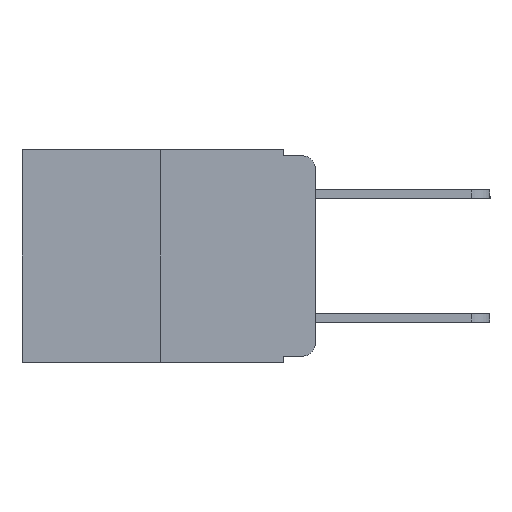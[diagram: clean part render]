
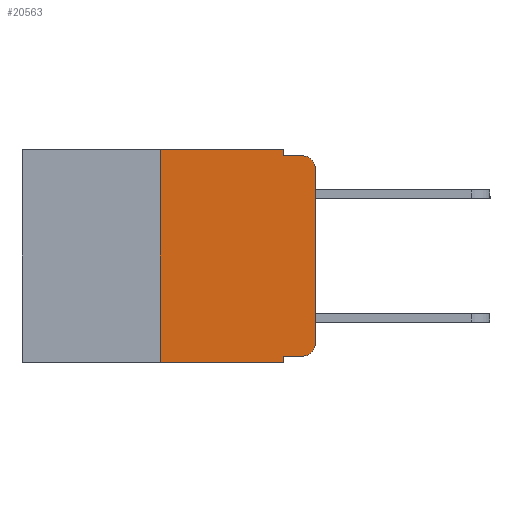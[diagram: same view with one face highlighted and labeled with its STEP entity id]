
A CAD part, left-side view. The second image highlights one B-rep face of the part: STEP entity #20563.
In plain terms, the highlighted planar face has unit normal (-1, 0, 0).
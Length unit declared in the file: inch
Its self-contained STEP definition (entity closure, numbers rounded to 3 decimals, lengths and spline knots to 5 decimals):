
#66 = AXIS2_PLACEMENT_3D ( 'NONE', #17826, #6917, #19643 ) ;
#268 = EDGE_CURVE ( 'NONE', #22494, #21428, #7474, .T. ) ;
#692 = CARTESIAN_POINT ( 'NONE',  ( 0., 0.02, -0.313 ) ) ;
#777 = LINE ( 'NONE', #12813, #20165 ) ;
#963 = DIRECTION ( 'NONE',  ( 0., 0., -1. ) ) ;
#1161 = EDGE_CURVE ( 'NONE', #17229, #2477, #17685, .T. ) ;
#1357 = FACE_OUTER_BOUND ( 'NONE', #18560, .T. ) ;
#1663 = CARTESIAN_POINT ( 'NONE',  ( 0., 0.25, 0. ) ) ;
#1903 = DIRECTION ( 'NONE',  ( 0., 0., -1. ) ) ;
#2344 = CARTESIAN_POINT ( 'NONE',  ( 0., 0.473, 0. ) ) ;
#2477 = VERTEX_POINT ( 'NONE', #13438 ) ;
#2492 = DIRECTION ( 'NONE',  ( 0., -1., 0. ) ) ;
#2836 = CARTESIAN_POINT ( 'NONE',  ( 0., 0.051, -0.01 ) ) ;
#3294 = CARTESIAN_POINT ( 'NONE',  ( 0., 0.25, 0. ) ) ;
#3795 = ORIENTED_EDGE ( 'NONE', *, *, #15224, .T. ) ;
#3817 = ORIENTED_EDGE ( 'NONE', *, *, #10504, .F. ) ;
#3820 = AXIS2_PLACEMENT_3D ( 'NONE', #692, #18908, #18046 ) ;
#4079 = CARTESIAN_POINT ( 'NONE',  ( 0., 0.02, -0.01 ) ) ;
#4166 = VERTEX_POINT ( 'NONE', #13520 ) ;
#4234 = VECTOR ( 'NONE', #13238, 39.37008 ) ;
#4329 = CARTESIAN_POINT ( 'NONE',  ( 0., 0.051, -0.333 ) ) ;
#4655 = ORIENTED_EDGE ( 'NONE', *, *, #16333, .F. ) ;
#4736 = VERTEX_POINT ( 'NONE', #11431 ) ;
#5077 = VERTEX_POINT ( 'NONE', #17805 ) ;
#5538 = ORIENTED_EDGE ( 'NONE', *, *, #10072, .T. ) ;
#5724 = CIRCLE ( 'NONE', #66, 0.02 ) ;
#5958 = LINE ( 'NONE', #2836, #10789 ) ;
#6004 = AXIS2_PLACEMENT_3D ( 'NONE', #22726, #11889, #963 ) ;
#6917 = DIRECTION ( 'NONE',  ( -1., 0., 0. ) ) ;
#6948 = VERTEX_POINT ( 'NONE', #10529 ) ;
#6951 = DIRECTION ( 'NONE',  ( 0., 0., 1. ) ) ;
#7245 = VERTEX_POINT ( 'NONE', #4079 ) ;
#7474 = CIRCLE ( 'NONE', #3820, 0.02 ) ;
#7503 = CARTESIAN_POINT ( 'NONE',  ( 0., 0.25, -0.343 ) ) ;
#7654 = DIRECTION ( 'NONE',  ( 0., 0., 1. ) ) ;
#7741 = VECTOR ( 'NONE', #2492, 39.37008 ) ;
#8998 = LINE ( 'NONE', #3294, #12116 ) ;
#9650 = DIRECTION ( 'NONE',  ( 0., 0., -1. ) ) ;
#10048 = PLANE ( 'NONE',  #6004 ) ;
#10072 = EDGE_CURVE ( 'NONE', #4736, #22494, #17439, .T. ) ;
#10504 = EDGE_CURVE ( 'NONE', #5077, #4166, #777, .T. ) ;
#10529 = CARTESIAN_POINT ( 'NONE',  ( 0., 0., -0.03 ) ) ;
#10643 = ORIENTED_EDGE ( 'NONE', *, *, #20434, .F. ) ;
#10789 = VECTOR ( 'NONE', #15574, 39.37008 ) ;
#11165 = ORIENTED_EDGE ( 'NONE', *, *, #12453, .T. ) ;
#11431 = CARTESIAN_POINT ( 'NONE',  ( 0., 0.051, -0.333 ) ) ;
#11889 = DIRECTION ( 'NONE',  ( 1., 0., 0. ) ) ;
#12116 = VECTOR ( 'NONE', #6951, 39.37008 ) ;
#12453 = EDGE_CURVE ( 'NONE', #21428, #6948, #16431, .T. ) ;
#12813 = CARTESIAN_POINT ( 'NONE',  ( 0., 0.051, 0. ) ) ;
#13238 = DIRECTION ( 'NONE',  ( 0., -1., 0. ) ) ;
#13334 = VECTOR ( 'NONE', #9650, 39.37008 ) ;
#13395 = VECTOR ( 'NONE', #18770, 39.37008 ) ;
#13438 = CARTESIAN_POINT ( 'NONE',  ( 0., 0.051, -0.343 ) ) ;
#13520 = CARTESIAN_POINT ( 'NONE',  ( 0., 0.051, -0.01 ) ) ;
#14058 = ORIENTED_EDGE ( 'NONE', *, *, #20413, .F. ) ;
#14644 = ORIENTED_EDGE ( 'NONE', *, *, #18916, .F. ) ;
#15108 = CARTESIAN_POINT ( 'NONE',  ( 0., 0.473, -0.343 ) ) ;
#15224 = EDGE_CURVE ( 'NONE', #6948, #7245, #5724, .T. ) ;
#15574 = DIRECTION ( 'NONE',  ( 0., -1., 0. ) ) ;
#16333 = EDGE_CURVE ( 'NONE', #4166, #7245, #5958, .T. ) ;
#16431 = LINE ( 'NONE', #16670, #20643 ) ;
#16670 = CARTESIAN_POINT ( 'NONE',  ( 0., 0., 0. ) ) ;
#17229 = VERTEX_POINT ( 'NONE', #7503 ) ;
#17439 = LINE ( 'NONE', #4329, #7741 ) ;
#17685 = LINE ( 'NONE', #15108, #13395 ) ;
#17805 = CARTESIAN_POINT ( 'NONE',  ( 0., 0.051, 0. ) ) ;
#17826 = CARTESIAN_POINT ( 'NONE',  ( 0., 0.02, -0.03 ) ) ;
#18046 = DIRECTION ( 'NONE',  ( 0., 0., -1. ) ) ;
#18560 = EDGE_LOOP ( 'NONE', ( #11165, #3795, #4655, #3817, #14058, #14644, #22819, #10643, #5538, #21169 ) ) ;
#18763 = LINE ( 'NONE', #2344, #4234 ) ;
#18770 = DIRECTION ( 'NONE',  ( 0., -1., 0. ) ) ;
#18908 = DIRECTION ( 'NONE',  ( -1., 0., 0. ) ) ;
#18916 = EDGE_CURVE ( 'NONE', #17229, #19515, #8998, .T. ) ;
#18999 = CARTESIAN_POINT ( 'NONE',  ( 0., 0., -0.313 ) ) ;
#19515 = VERTEX_POINT ( 'NONE', #1663 ) ;
#19643 = DIRECTION ( 'NONE',  ( 0., 0., -1. ) ) ;
#20165 = VECTOR ( 'NONE', #1903, 39.37008 ) ;
#20413 = EDGE_CURVE ( 'NONE', #19515, #5077, #18763, .T. ) ;
#20434 = EDGE_CURVE ( 'NONE', #4736, #2477, #22951, .T. ) ;
#20554 = CARTESIAN_POINT ( 'NONE',  ( 0., 0.051, 0. ) ) ;
#20563 = ADVANCED_FACE ( 'NONE', ( #1357 ), #10048, .F. ) ;
#20643 = VECTOR ( 'NONE', #7654, 39.37008 ) ;
#21169 = ORIENTED_EDGE ( 'NONE', *, *, #268, .T. ) ;
#21428 = VERTEX_POINT ( 'NONE', #18999 ) ;
#22298 = CARTESIAN_POINT ( 'NONE',  ( 0., 0.02, -0.333 ) ) ;
#22494 = VERTEX_POINT ( 'NONE', #22298 ) ;
#22726 = CARTESIAN_POINT ( 'NONE',  ( 0., 0.473, 0. ) ) ;
#22819 = ORIENTED_EDGE ( 'NONE', *, *, #1161, .T. ) ;
#22951 = LINE ( 'NONE', #20554, #13334 ) ;
